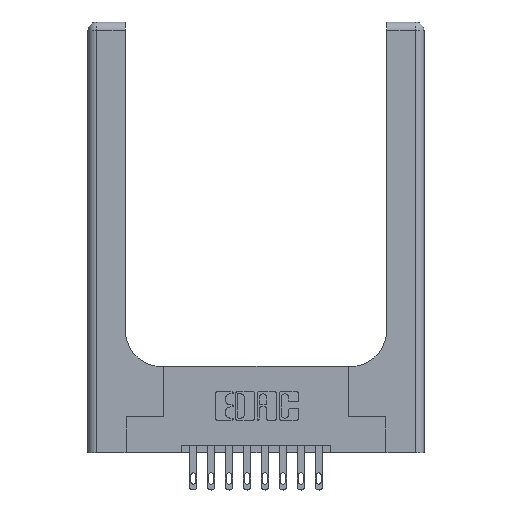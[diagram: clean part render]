
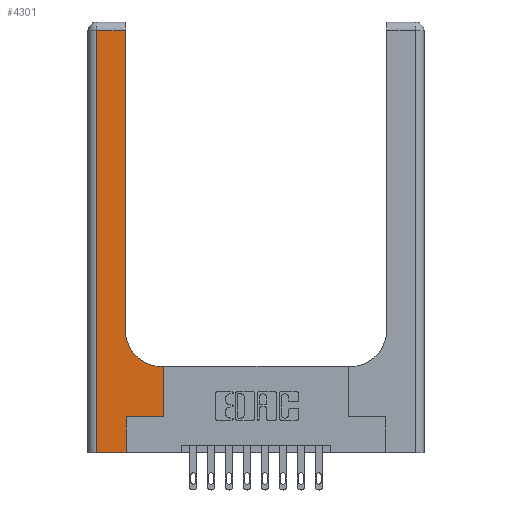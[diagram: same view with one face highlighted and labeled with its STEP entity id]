
A CAD part, top view. The second image highlights one B-rep face of the part: STEP entity #4301.
In plain terms, the highlighted planar face has unit normal (0, 0, 1).
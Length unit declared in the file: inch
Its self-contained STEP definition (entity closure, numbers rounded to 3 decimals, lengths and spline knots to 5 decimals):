
#106 = EDGE_CURVE ( 'NONE', #12288, #9125, #1347, .T. ) ;
#113 = DIRECTION ( 'NONE',  ( 0., -1., 0. ) ) ;
#381 = CARTESIAN_POINT ( 'NONE',  ( 0.26, 3., 0.37 ) ) ;
#390 = VERTEX_POINT ( 'NONE', #994 ) ;
#432 = VERTEX_POINT ( 'NONE', #1426 ) ;
#434 = DIRECTION ( 'NONE',  ( 1., 0., 0. ) ) ;
#706 = DIRECTION ( 'NONE',  ( 0., 0., -1. ) ) ;
#939 = VECTOR ( 'NONE', #12694, 39.37008 ) ;
#994 = CARTESIAN_POINT ( 'NONE',  ( 0.26, 2.94, 0.37 ) ) ;
#1347 = LINE ( 'NONE', #2613, #12380 ) ;
#1426 = CARTESIAN_POINT ( 'NONE',  ( 0.51, 0.6, 0.37 ) ) ;
#1855 = PLANE ( 'NONE',  #9818 ) ;
#1914 = VECTOR ( 'NONE', #113, 39.37008 ) ;
#2099 = VECTOR ( 'NONE', #15050, 39.37008 ) ;
#2354 = CARTESIAN_POINT ( 'NONE',  ( 0.265, 0., 0.37 ) ) ;
#2587 = LINE ( 'NONE', #10652, #10835 ) ;
#2595 = CARTESIAN_POINT ( 'NONE',  ( 0.06, 3., 0.37 ) ) ;
#2600 = EDGE_CURVE ( 'NONE', #432, #7444, #11559, .T. ) ;
#2613 = CARTESIAN_POINT ( 'NONE',  ( 0.528, 0.25, 0.37 ) ) ;
#3205 = ORIENTED_EDGE ( 'NONE', *, *, #5346, .T. ) ;
#3239 = EDGE_LOOP ( 'NONE', ( #12325, #11008, #4278, #3205, #12172, #5634, #15182, #5740, #8441 ) ) ;
#4278 = ORIENTED_EDGE ( 'NONE', *, *, #10919, .T. ) ;
#4301 = ADVANCED_FACE ( 'NONE', ( #13672 ), #1855, .F. ) ;
#4391 = DIRECTION ( 'NONE',  ( 1., 0., 0. ) ) ;
#4714 = CARTESIAN_POINT ( 'NONE',  ( 0.265, 0.25, 0.37 ) ) ;
#5175 = VERTEX_POINT ( 'NONE', #4714 ) ;
#5346 = EDGE_CURVE ( 'NONE', #5488, #12517, #7649, .T. ) ;
#5424 = DIRECTION ( 'NONE',  ( -1., 0., 0. ) ) ;
#5488 = VERTEX_POINT ( 'NONE', #10342 ) ;
#5622 = VECTOR ( 'NONE', #434, 39.37008 ) ;
#5634 = ORIENTED_EDGE ( 'NONE', *, *, #5802, .T. ) ;
#5740 = ORIENTED_EDGE ( 'NONE', *, *, #13439, .T. ) ;
#5802 = EDGE_CURVE ( 'NONE', #5175, #12288, #13798, .T. ) ;
#5810 = CARTESIAN_POINT ( 'NONE',  ( 0.528, 0.25, 0.37 ) ) ;
#5838 = LINE ( 'NONE', #14101, #13255 ) ;
#7181 = DIRECTION ( 'NONE',  ( -1., 0., 0. ) ) ;
#7444 = VERTEX_POINT ( 'NONE', #10573 ) ;
#7649 = LINE ( 'NONE', #11145, #5622 ) ;
#7931 = CARTESIAN_POINT ( 'NONE',  ( 0.528, 0.6, 0.37 ) ) ;
#8182 = DIRECTION ( 'NONE',  ( -1., 0., 0. ) ) ;
#8333 = VECTOR ( 'NONE', #9246, 39.37008 ) ;
#8441 = ORIENTED_EDGE ( 'NONE', *, *, #2600, .T. ) ;
#8723 = CARTESIAN_POINT ( 'NONE',  ( 0.265, 0., 0.37 ) ) ;
#8836 = AXIS2_PLACEMENT_3D ( 'NONE', #14818, #13789, #4391 ) ;
#9125 = VERTEX_POINT ( 'NONE', #7931 ) ;
#9246 = DIRECTION ( 'NONE',  ( 0., 1., 0. ) ) ;
#9818 = AXIS2_PLACEMENT_3D ( 'NONE', #10299, #706, #5424 ) ;
#10299 = CARTESIAN_POINT ( 'NONE',  ( 0., 3., 0.37 ) ) ;
#10342 = CARTESIAN_POINT ( 'NONE',  ( 0.06, 0., 0.37 ) ) ;
#10513 = CARTESIAN_POINT ( 'NONE',  ( 0.265, 0.25, 0.37 ) ) ;
#10573 = CARTESIAN_POINT ( 'NONE',  ( 0.26, 0.85, 0.37 ) ) ;
#10652 = CARTESIAN_POINT ( 'NONE',  ( 0., 2.94, 0.37 ) ) ;
#10800 = LINE ( 'NONE', #2595, #1914 ) ;
#10835 = VECTOR ( 'NONE', #7181, 39.37008 ) ;
#10919 = EDGE_CURVE ( 'NONE', #13776, #5488, #10800, .T. ) ;
#11008 = ORIENTED_EDGE ( 'NONE', *, *, #11477, .T. ) ;
#11058 = CARTESIAN_POINT ( 'NONE',  ( 0.06, 2.94, 0.37 ) ) ;
#11145 = CARTESIAN_POINT ( 'NONE',  ( 0., 0., 0.37 ) ) ;
#11477 = EDGE_CURVE ( 'NONE', #390, #13776, #2587, .T. ) ;
#11559 = CIRCLE ( 'NONE', #8836, 0.25 ) ;
#11935 = EDGE_CURVE ( 'NONE', #12517, #5175, #12741, .T. ) ;
#12068 = DIRECTION ( 'NONE',  ( 0., 1., 0. ) ) ;
#12172 = ORIENTED_EDGE ( 'NONE', *, *, #11935, .T. ) ;
#12288 = VERTEX_POINT ( 'NONE', #5810 ) ;
#12325 = ORIENTED_EDGE ( 'NONE', *, *, #13519, .T. ) ;
#12380 = VECTOR ( 'NONE', #12068, 39.37008 ) ;
#12517 = VERTEX_POINT ( 'NONE', #8723 ) ;
#12694 = DIRECTION ( 'NONE',  ( 1., 0., 0. ) ) ;
#12741 = LINE ( 'NONE', #2354, #8333 ) ;
#13255 = VECTOR ( 'NONE', #8182, 39.37008 ) ;
#13439 = EDGE_CURVE ( 'NONE', #9125, #432, #5838, .T. ) ;
#13519 = EDGE_CURVE ( 'NONE', #7444, #390, #14607, .T. ) ;
#13672 = FACE_OUTER_BOUND ( 'NONE', #3239, .T. ) ;
#13776 = VERTEX_POINT ( 'NONE', #11058 ) ;
#13789 = DIRECTION ( 'NONE',  ( 0., 0., -1. ) ) ;
#13798 = LINE ( 'NONE', #10513, #939 ) ;
#14101 = CARTESIAN_POINT ( 'NONE',  ( 0.26, 0.6, 0.37 ) ) ;
#14607 = LINE ( 'NONE', #381, #2099 ) ;
#14818 = CARTESIAN_POINT ( 'NONE',  ( 0.51, 0.85, 0.37 ) ) ;
#15050 = DIRECTION ( 'NONE',  ( 0., 1., 0. ) ) ;
#15182 = ORIENTED_EDGE ( 'NONE', *, *, #106, .T. ) ;
